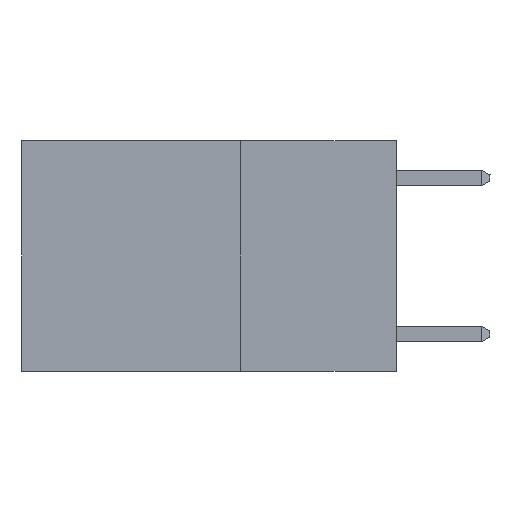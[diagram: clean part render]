
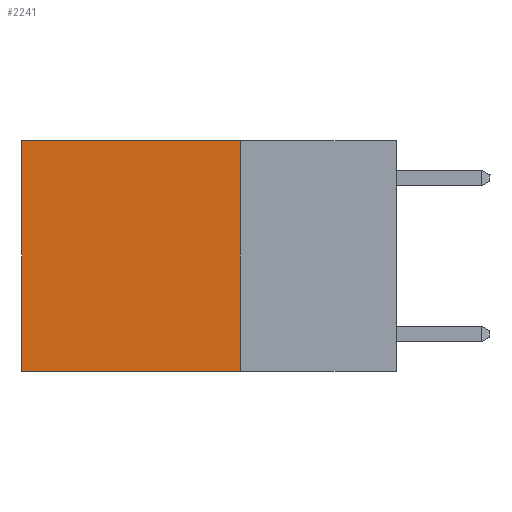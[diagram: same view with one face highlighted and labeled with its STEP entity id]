
A CAD part, left-side view. The second image highlights one B-rep face of the part: STEP entity #2241.
In plain terms, the highlighted planar face has unit normal (-1, 0, 0).
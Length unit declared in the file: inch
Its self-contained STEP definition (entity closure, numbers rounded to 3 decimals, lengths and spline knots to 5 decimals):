
#223 = EDGE_CURVE ( 'NONE', #9910, #5608, #4981, .T. ) ;
#310 = FACE_OUTER_BOUND ( 'NONE', #7799, .T. ) ;
#505 = DIRECTION ( 'NONE',  ( 0., 1., 0. ) ) ;
#521 = VERTEX_POINT ( 'NONE', #7056 ) ;
#1305 = ORIENTED_EDGE ( 'NONE', *, *, #223, .F. ) ;
#1724 = CARTESIAN_POINT ( 'NONE',  ( 0.2625, 0.25, -0.37 ) ) ;
#1776 = LINE ( 'NONE', #8703, #2069 ) ;
#2069 = VECTOR ( 'NONE', #4065, 39.37008 ) ;
#2241 = ADVANCED_FACE ( 'NONE', ( #310 ), #3448, .F. ) ;
#2455 = EDGE_CURVE ( 'NONE', #9910, #7552, #1776, .T. ) ;
#2609 = AXIS2_PLACEMENT_3D ( 'NONE', #5791, #4245, #9637 ) ;
#3438 = ORIENTED_EDGE ( 'NONE', *, *, #10019, .T. ) ;
#3448 = PLANE ( 'NONE',  #2609 ) ;
#3686 = ORIENTED_EDGE ( 'NONE', *, *, #2455, .T. ) ;
#4065 = DIRECTION ( 'NONE',  ( 0., 1., 0. ) ) ;
#4245 = DIRECTION ( 'NONE',  ( 1., 0., 0. ) ) ;
#4592 = EDGE_CURVE ( 'NONE', #5608, #521, #9171, .T. ) ;
#4713 = DIRECTION ( 'NONE',  ( 0., 0., -1. ) ) ;
#4883 = CARTESIAN_POINT ( 'NONE',  ( 0.2625, 0.6, 0. ) ) ;
#4981 = LINE ( 'NONE', #10185, #8859 ) ;
#5587 = CARTESIAN_POINT ( 'NONE',  ( 0.2625, 0.6, 0. ) ) ;
#5608 = VERTEX_POINT ( 'NONE', #10107 ) ;
#5791 = CARTESIAN_POINT ( 'NONE',  ( 0.2625, 0.25, 0. ) ) ;
#6711 = LINE ( 'NONE', #5587, #8531 ) ;
#7056 = CARTESIAN_POINT ( 'NONE',  ( 0.2625, 0.6, -0.37 ) ) ;
#7150 = VECTOR ( 'NONE', #505, 39.37008 ) ;
#7552 = VERTEX_POINT ( 'NONE', #4883 ) ;
#7799 = EDGE_LOOP ( 'NONE', ( #3438, #9607, #1305, #3686 ) ) ;
#7879 = DIRECTION ( 'NONE',  ( 0., 0., -1. ) ) ;
#8531 = VECTOR ( 'NONE', #7879, 39.37008 ) ;
#8703 = CARTESIAN_POINT ( 'NONE',  ( 0.2625, 0.25, 0. ) ) ;
#8859 = VECTOR ( 'NONE', #4713, 39.37008 ) ;
#9171 = LINE ( 'NONE', #1724, #7150 ) ;
#9607 = ORIENTED_EDGE ( 'NONE', *, *, #4592, .F. ) ;
#9637 = DIRECTION ( 'NONE',  ( 0., 0., -1. ) ) ;
#9910 = VERTEX_POINT ( 'NONE', #10084 ) ;
#10019 = EDGE_CURVE ( 'NONE', #7552, #521, #6711, .T. ) ;
#10084 = CARTESIAN_POINT ( 'NONE',  ( 0.2625, 0.25, 0. ) ) ;
#10107 = CARTESIAN_POINT ( 'NONE',  ( 0.2625, 0.25, -0.37 ) ) ;
#10185 = CARTESIAN_POINT ( 'NONE',  ( 0.2625, 0.25, 0. ) ) ;
